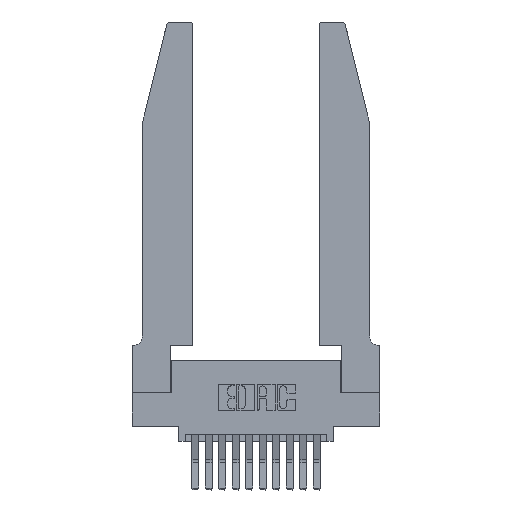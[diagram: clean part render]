
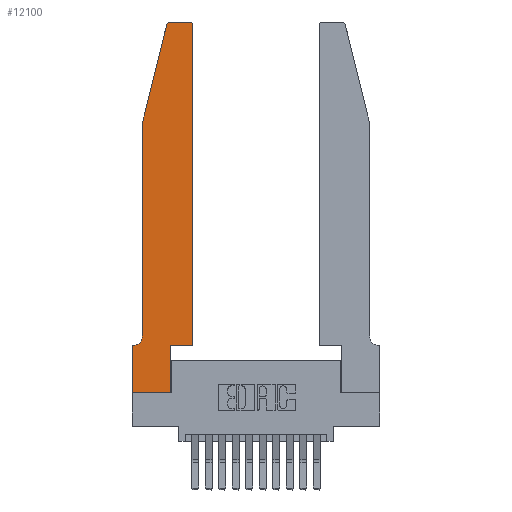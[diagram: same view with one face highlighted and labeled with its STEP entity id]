
A CAD part, top view. The second image highlights one B-rep face of the part: STEP entity #12100.
In plain terms, the highlighted planar face has unit normal (0, 0, 1).
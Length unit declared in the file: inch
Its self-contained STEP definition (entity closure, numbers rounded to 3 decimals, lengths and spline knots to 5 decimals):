
#202 = CARTESIAN_POINT ( 'NONE',  ( 0.2865, 0.35, 0.37 ) ) ;
#274 = EDGE_CURVE ( 'NONE', #3404, #14329, #12438, .T. ) ;
#484 = CIRCLE ( 'NONE', #16671, 0.03 ) ;
#562 = EDGE_CURVE ( 'NONE', #14329, #10706, #2556, .T. ) ;
#695 = VECTOR ( 'NONE', #14713, 39.37008 ) ;
#1334 = ORIENTED_EDGE ( 'NONE', *, *, #10196, .T. ) ;
#1507 = EDGE_CURVE ( 'NONE', #11047, #4543, #4950, .T. ) ;
#1726 = VERTEX_POINT ( 'NONE', #202 ) ;
#1760 = EDGE_LOOP ( 'NONE', ( #7681, #12466, #7819, #7396, #8685, #3120, #1334, #11996, #9605, #3920, #11034, #14592 ) ) ;
#1782 = CARTESIAN_POINT ( 'NONE',  ( 0.284, 2.75, 0.37 ) ) ;
#1854 = CARTESIAN_POINT ( 'NONE',  ( 0., 0.35, 0.37 ) ) ;
#1993 = CARTESIAN_POINT ( 'NONE',  ( 0.0755, 2., 0.37 ) ) ;
#2055 = EDGE_CURVE ( 'NONE', #9429, #9002, #14421, .T. ) ;
#2233 = CARTESIAN_POINT ( 'NONE',  ( 0.2865, 0.35, 0.37 ) ) ;
#2348 = VECTOR ( 'NONE', #5830, 39.37008 ) ;
#2556 = CIRCLE ( 'NONE', #7224, 0.03 ) ;
#2658 = EDGE_CURVE ( 'NONE', #16044, #2969, #16548, .T. ) ;
#2969 = VERTEX_POINT ( 'NONE', #16097 ) ;
#3045 = CARTESIAN_POINT ( 'NONE',  ( 0.4505, 0.35, 0.37 ) ) ;
#3120 = ORIENTED_EDGE ( 'NONE', *, *, #1507, .T. ) ;
#3404 = VERTEX_POINT ( 'NONE', #12236 ) ;
#3581 = EDGE_CURVE ( 'NONE', #9002, #11131, #14750, .T. ) ;
#3920 = ORIENTED_EDGE ( 'NONE', *, *, #13895, .T. ) ;
#4184 = CARTESIAN_POINT ( 'NONE',  ( 0.4205, 2.75, 0.37 ) ) ;
#4434 = VECTOR ( 'NONE', #15228, 39.37008 ) ;
#4515 = VECTOR ( 'NONE', #15796, 39.37008 ) ;
#4543 = VERTEX_POINT ( 'NONE', #1854 ) ;
#4545 = CARTESIAN_POINT ( 'NONE',  ( 0., 0., 0.37 ) ) ;
#4741 = FACE_OUTER_BOUND ( 'NONE', #1760, .T. ) ;
#4950 = LINE ( 'NONE', #11307, #4515 ) ;
#5185 = PLANE ( 'NONE',  #6613 ) ;
#5658 = DIRECTION ( 'NONE',  ( 1., 0., 0. ) ) ;
#5671 = CARTESIAN_POINT ( 'NONE',  ( 0.4505, 2.72, 0.37 ) ) ;
#5830 = DIRECTION ( 'NONE',  ( 0., 1., 0. ) ) ;
#6181 = DIRECTION ( 'NONE',  ( 0., 0., -1. ) ) ;
#6321 = VECTOR ( 'NONE', #8903, 39.37008 ) ;
#6346 = VECTOR ( 'NONE', #14717, 39.37008 ) ;
#6413 = DIRECTION ( 'NONE',  ( 0., 0., 1. ) ) ;
#6613 = AXIS2_PLACEMENT_3D ( 'NONE', #14190, #15437, #7740 ) ;
#6761 = LINE ( 'NONE', #2233, #9826 ) ;
#6841 = CARTESIAN_POINT ( 'NONE',  ( 0.4505, 0.35, 0.37 ) ) ;
#7007 = CARTESIAN_POINT ( 'NONE',  ( 0., 0., 0.37 ) ) ;
#7035 = CARTESIAN_POINT ( 'NONE',  ( 0., 0., 0.37 ) ) ;
#7224 = AXIS2_PLACEMENT_3D ( 'NONE', #12650, #14257, #5658 ) ;
#7304 = EDGE_CURVE ( 'NONE', #10706, #7767, #8437, .T. ) ;
#7396 = ORIENTED_EDGE ( 'NONE', *, *, #3581, .T. ) ;
#7681 = ORIENTED_EDGE ( 'NONE', *, *, #7304, .T. ) ;
#7698 = AXIS2_PLACEMENT_3D ( 'NONE', #13904, #6181, #15148 ) ;
#7740 = DIRECTION ( 'NONE',  ( 1., 0., 0. ) ) ;
#7767 = VERTEX_POINT ( 'NONE', #1782 ) ;
#7819 = ORIENTED_EDGE ( 'NONE', *, *, #2055, .T. ) ;
#8437 = LINE ( 'NONE', #16099, #14862 ) ;
#8685 = ORIENTED_EDGE ( 'NONE', *, *, #15210, .T. ) ;
#8884 = DIRECTION ( 'NONE',  ( 0., 1., 0. ) ) ;
#8903 = DIRECTION ( 'NONE',  ( 1., 0., 0. ) ) ;
#9002 = VERTEX_POINT ( 'NONE', #1993 ) ;
#9332 = EDGE_CURVE ( 'NONE', #7767, #9429, #484, .T. ) ;
#9429 = VERTEX_POINT ( 'NONE', #15496 ) ;
#9552 = CIRCLE ( 'NONE', #7698, 0.07 ) ;
#9605 = ORIENTED_EDGE ( 'NONE', *, *, #12452, .T. ) ;
#9826 = VECTOR ( 'NONE', #8884, 39.37008 ) ;
#10133 = CARTESIAN_POINT ( 'NONE',  ( 0.0055, 0.35, 0.37 ) ) ;
#10196 = EDGE_CURVE ( 'NONE', #4543, #16044, #12816, .T. ) ;
#10706 = VERTEX_POINT ( 'NONE', #4184 ) ;
#10940 = DIRECTION ( 'NONE',  ( 1., 0., 0. ) ) ;
#11034 = ORIENTED_EDGE ( 'NONE', *, *, #274, .T. ) ;
#11047 = VERTEX_POINT ( 'NONE', #10133 ) ;
#11131 = VERTEX_POINT ( 'NONE', #16621 ) ;
#11307 = CARTESIAN_POINT ( 'NONE',  ( 0.0755, 0.35, 0.37 ) ) ;
#11996 = ORIENTED_EDGE ( 'NONE', *, *, #2658, .T. ) ;
#12100 = ADVANCED_FACE ( 'NONE', ( #4741 ), #5185, .T. ) ;
#12236 = CARTESIAN_POINT ( 'NONE',  ( 0.4505, 0.35, 0.37 ) ) ;
#12438 = LINE ( 'NONE', #6841, #2348 ) ;
#12452 = EDGE_CURVE ( 'NONE', #2969, #1726, #6761, .T. ) ;
#12466 = ORIENTED_EDGE ( 'NONE', *, *, #9332, .T. ) ;
#12650 = CARTESIAN_POINT ( 'NONE',  ( 0.4205, 2.72, 0.37 ) ) ;
#12773 = VECTOR ( 'NONE', #10940, 39.37008 ) ;
#12816 = LINE ( 'NONE', #7007, #6346 ) ;
#13895 = EDGE_CURVE ( 'NONE', #1726, #3404, #16132, .T. ) ;
#13904 = CARTESIAN_POINT ( 'NONE',  ( 0.0055, 0.42, 0.37 ) ) ;
#14150 = CARTESIAN_POINT ( 'NONE',  ( 0.284, 2.72, 0.37 ) ) ;
#14190 = CARTESIAN_POINT ( 'NONE',  ( 0., 0.35, 0.37 ) ) ;
#14257 = DIRECTION ( 'NONE',  ( 0., 0., 1. ) ) ;
#14329 = VERTEX_POINT ( 'NONE', #5671 ) ;
#14421 = LINE ( 'NONE', #16169, #695 ) ;
#14592 = ORIENTED_EDGE ( 'NONE', *, *, #562, .T. ) ;
#14713 = DIRECTION ( 'NONE',  ( -0.239, -0.971, 0. ) ) ;
#14717 = DIRECTION ( 'NONE',  ( 0., -1., 0. ) ) ;
#14750 = LINE ( 'NONE', #16491, #4434 ) ;
#14862 = VECTOR ( 'NONE', #16152, 39.37008 ) ;
#15148 = DIRECTION ( 'NONE',  ( -1., 0., 0. ) ) ;
#15210 = EDGE_CURVE ( 'NONE', #11131, #11047, #9552, .T. ) ;
#15228 = DIRECTION ( 'NONE',  ( 0., -1., 0. ) ) ;
#15398 = DIRECTION ( 'NONE',  ( 1., 0., 0. ) ) ;
#15437 = DIRECTION ( 'NONE',  ( 0., 0., 1. ) ) ;
#15496 = CARTESIAN_POINT ( 'NONE',  ( 0.25487, 2.72718, 0.37 ) ) ;
#15796 = DIRECTION ( 'NONE',  ( -1., 0., 0. ) ) ;
#16044 = VERTEX_POINT ( 'NONE', #7035 ) ;
#16097 = CARTESIAN_POINT ( 'NONE',  ( 0.2865, 0., 0.37 ) ) ;
#16099 = CARTESIAN_POINT ( 'NONE',  ( 0.2605, 2.75, 0.37 ) ) ;
#16132 = LINE ( 'NONE', #3045, #12773 ) ;
#16152 = DIRECTION ( 'NONE',  ( -1., 0., 0. ) ) ;
#16169 = CARTESIAN_POINT ( 'NONE',  ( 0.0755, 2., 0.37 ) ) ;
#16491 = CARTESIAN_POINT ( 'NONE',  ( 0.0755, 2., 0.37 ) ) ;
#16548 = LINE ( 'NONE', #4545, #6321 ) ;
#16621 = CARTESIAN_POINT ( 'NONE',  ( 0.0755, 0.42, 0.37 ) ) ;
#16671 = AXIS2_PLACEMENT_3D ( 'NONE', #14150, #6413, #15398 ) ;
